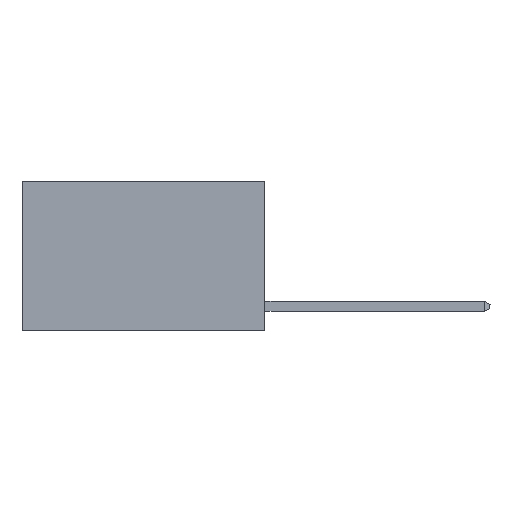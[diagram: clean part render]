
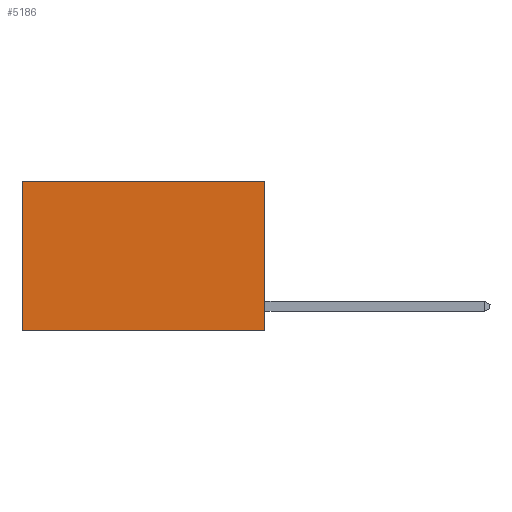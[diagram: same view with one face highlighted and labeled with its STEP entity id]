
A CAD part, left-side view. The second image highlights one B-rep face of the part: STEP entity #5186.
In plain terms, the highlighted planar face has unit normal (-1, 0, 0).
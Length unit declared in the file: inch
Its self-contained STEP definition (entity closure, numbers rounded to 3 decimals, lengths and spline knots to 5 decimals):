
#98 = CARTESIAN_POINT ( 'NONE',  ( 0.2625, 0., 0. ) ) ;
#226 = VERTEX_POINT ( 'NONE', #11930 ) ;
#679 = CARTESIAN_POINT ( 'NONE',  ( 0.2625, 0., 0. ) ) ;
#796 = DIRECTION ( 'NONE',  ( 0., 0., -1. ) ) ;
#1334 = ORIENTED_EDGE ( 'NONE', *, *, #11865, .T. ) ;
#2009 = DIRECTION ( 'NONE',  ( 1., 0., 0. ) ) ;
#2542 = EDGE_CURVE ( 'NONE', #7681, #4880, #12225, .T. ) ;
#2561 = VECTOR ( 'NONE', #13629, 39.37008 ) ;
#2565 = ORIENTED_EDGE ( 'NONE', *, *, #7479, .F. ) ;
#3352 = VECTOR ( 'NONE', #8429, 39.37008 ) ;
#4880 = VERTEX_POINT ( 'NONE', #12510 ) ;
#5186 = ADVANCED_FACE ( 'NONE', ( #6912 ), #13138, .F. ) ;
#5899 = CARTESIAN_POINT ( 'NONE',  ( 0.2625, 0., -0.37 ) ) ;
#6119 = AXIS2_PLACEMENT_3D ( 'NONE', #7069, #2009, #796 ) ;
#6335 = LINE ( 'NONE', #13705, #2561 ) ;
#6912 = FACE_OUTER_BOUND ( 'NONE', #9561, .T. ) ;
#7069 = CARTESIAN_POINT ( 'NONE',  ( 0.2625, 0., 0. ) ) ;
#7433 = ORIENTED_EDGE ( 'NONE', *, *, #2542, .F. ) ;
#7479 = EDGE_CURVE ( 'NONE', #15595, #7681, #9133, .T. ) ;
#7681 = VERTEX_POINT ( 'NONE', #5899 ) ;
#7872 = EDGE_CURVE ( 'NONE', #226, #4880, #12841, .T. ) ;
#8062 = CARTESIAN_POINT ( 'NONE',  ( 0.2625, 0.6, 0. ) ) ;
#8237 = DIRECTION ( 'NONE',  ( 0., 0., -1. ) ) ;
#8429 = DIRECTION ( 'NONE',  ( 0., 1., 0. ) ) ;
#9133 = LINE ( 'NONE', #679, #11864 ) ;
#9303 = ORIENTED_EDGE ( 'NONE', *, *, #7872, .T. ) ;
#9561 = EDGE_LOOP ( 'NONE', ( #9303, #7433, #2565, #1334 ) ) ;
#11078 = CARTESIAN_POINT ( 'NONE',  ( 0.2625, 0., -0.37 ) ) ;
#11864 = VECTOR ( 'NONE', #8237, 39.37008 ) ;
#11865 = EDGE_CURVE ( 'NONE', #15595, #226, #6335, .T. ) ;
#11930 = CARTESIAN_POINT ( 'NONE',  ( 0.2625, 0.6, 0. ) ) ;
#12225 = LINE ( 'NONE', #11078, #3352 ) ;
#12510 = CARTESIAN_POINT ( 'NONE',  ( 0.2625, 0.6, -0.37 ) ) ;
#12841 = LINE ( 'NONE', #8062, #13174 ) ;
#13138 = PLANE ( 'NONE',  #6119 ) ;
#13174 = VECTOR ( 'NONE', #14081, 39.37008 ) ;
#13629 = DIRECTION ( 'NONE',  ( 0., 1., 0. ) ) ;
#13705 = CARTESIAN_POINT ( 'NONE',  ( 0.2625, 0., 0. ) ) ;
#14081 = DIRECTION ( 'NONE',  ( 0., 0., -1. ) ) ;
#15595 = VERTEX_POINT ( 'NONE', #98 ) ;
